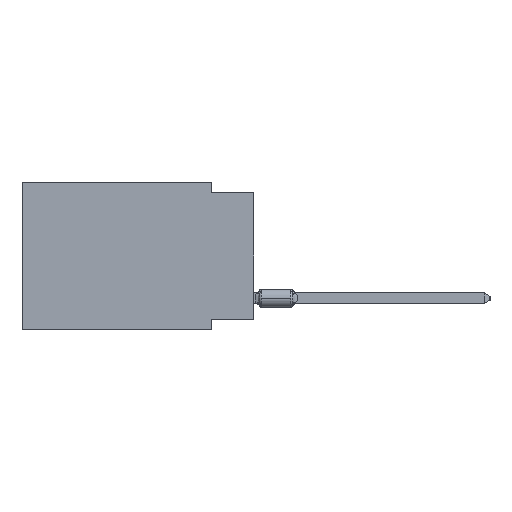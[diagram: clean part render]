
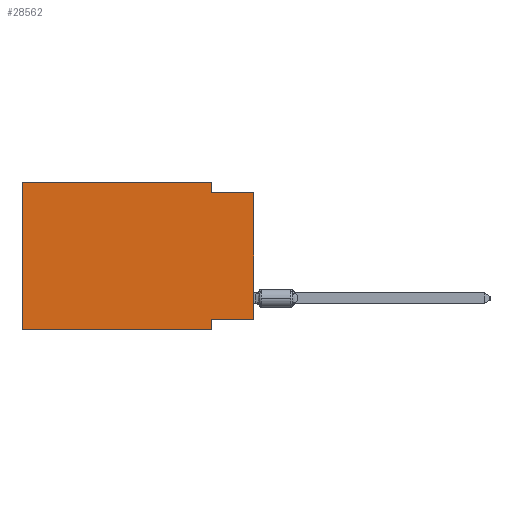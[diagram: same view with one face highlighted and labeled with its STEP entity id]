
A CAD part, left-side view. The second image highlights one B-rep face of the part: STEP entity #28562.
In plain terms, the highlighted planar face has unit normal (-1, 0, 0).
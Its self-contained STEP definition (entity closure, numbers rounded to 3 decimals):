
#42 = CARTESIAN_POINT ( 'NONE',  ( 0., 2.54, -8.89 ) ) ;
#937 = VECTOR ( 'NONE', #26357, 1000. ) ;
#982 = VECTOR ( 'NONE', #10857, 1000. ) ;
#1257 = EDGE_CURVE ( 'NONE', #8671, #54675, #59619, .T. ) ;
#1369 = LINE ( 'NONE', #26887, #47268 ) ;
#2557 = DIRECTION ( 'NONE',  ( 0., -1., 0. ) ) ;
#3318 = ORIENTED_EDGE ( 'NONE', *, *, #5943, .F. ) ;
#3636 = VERTEX_POINT ( 'NONE', #57415 ) ;
#4593 = CARTESIAN_POINT ( 'NONE',  ( 0., 2.54, 0. ) ) ;
#5943 = EDGE_CURVE ( 'NONE', #54675, #44059, #8694, .T. ) ;
#8671 = VERTEX_POINT ( 'NONE', #29459 ) ;
#8694 = LINE ( 'NONE', #29465, #54876 ) ;
#10195 = DIRECTION ( 'NONE',  ( 0., 1., 0. ) ) ;
#10857 = DIRECTION ( 'NONE',  ( 0., -1., 0. ) ) ;
#11293 = DIRECTION ( 'NONE',  ( 0., 0., 1. ) ) ;
#16132 = ORIENTED_EDGE ( 'NONE', *, *, #48546, .F. ) ;
#16175 = LINE ( 'NONE', #36650, #50894 ) ;
#16806 = DIRECTION ( 'NONE',  ( 0., 0., -1. ) ) ;
#19431 = VECTOR ( 'NONE', #11293, 1000. ) ;
#19963 = LINE ( 'NONE', #39179, #43681 ) ;
#20591 = CARTESIAN_POINT ( 'NONE',  ( 0., 2.54, -8.255 ) ) ;
#20739 = CARTESIAN_POINT ( 'NONE',  ( 0., 0., -8.255 ) ) ;
#21193 = AXIS2_PLACEMENT_3D ( 'NONE', #35976, #40442, #39469 ) ;
#21738 = CARTESIAN_POINT ( 'NONE',  ( 0., 13.97, -8.89 ) ) ;
#24330 = EDGE_LOOP ( 'NONE', ( #51633, #59758, #40295, #3318, #35253, #30114, #16132, #40734 ) ) ;
#25411 = PLANE ( 'NONE',  #21193 ) ;
#25545 = EDGE_CURVE ( 'NONE', #44059, #44435, #19963, .T. ) ;
#26357 = DIRECTION ( 'NONE',  ( 0., 0., 1. ) ) ;
#26548 = CARTESIAN_POINT ( 'NONE',  ( 0., 2.54, -0.635 ) ) ;
#26887 = CARTESIAN_POINT ( 'NONE',  ( 0., 0., -0.635 ) ) ;
#28562 = ADVANCED_FACE ( 'NONE', ( #44596 ), #25411, .F. ) ;
#29459 = CARTESIAN_POINT ( 'NONE',  ( 0., 13.97, -8.89 ) ) ;
#29465 = CARTESIAN_POINT ( 'NONE',  ( 0., 13.97, 0. ) ) ;
#29962 = VECTOR ( 'NONE', #10195, 1000. ) ;
#30114 = ORIENTED_EDGE ( 'NONE', *, *, #44304, .T. ) ;
#35253 = ORIENTED_EDGE ( 'NONE', *, *, #1257, .F. ) ;
#35976 = CARTESIAN_POINT ( 'NONE',  ( 0., 13.97, 0. ) ) ;
#36650 = CARTESIAN_POINT ( 'NONE',  ( 0., 2.54, -8.89 ) ) ;
#37870 = EDGE_CURVE ( 'NONE', #56214, #62409, #40573, .T. ) ;
#39179 = CARTESIAN_POINT ( 'NONE',  ( 0., 2.54, 0. ) ) ;
#39469 = DIRECTION ( 'NONE',  ( 0., 0., -1. ) ) ;
#40067 = CARTESIAN_POINT ( 'NONE',  ( 0., 0., -8.255 ) ) ;
#40295 = ORIENTED_EDGE ( 'NONE', *, *, #25545, .F. ) ;
#40442 = DIRECTION ( 'NONE',  ( 1., 0., 0. ) ) ;
#40573 = LINE ( 'NONE', #20739, #29962 ) ;
#40734 = ORIENTED_EDGE ( 'NONE', *, *, #37870, .F. ) ;
#42181 = CARTESIAN_POINT ( 'NONE',  ( 0., 13.97, 0. ) ) ;
#42943 = EDGE_CURVE ( 'NONE', #56214, #3636, #44541, .T. ) ;
#43681 = VECTOR ( 'NONE', #58987, 1000. ) ;
#44059 = VERTEX_POINT ( 'NONE', #4593 ) ;
#44304 = EDGE_CURVE ( 'NONE', #8671, #61014, #55639, .T. ) ;
#44435 = VERTEX_POINT ( 'NONE', #26548 ) ;
#44541 = LINE ( 'NONE', #44886, #19431 ) ;
#44596 = FACE_OUTER_BOUND ( 'NONE', #24330, .T. ) ;
#44886 = CARTESIAN_POINT ( 'NONE',  ( 0., 0., 0. ) ) ;
#47268 = VECTOR ( 'NONE', #2557, 1000. ) ;
#48546 = EDGE_CURVE ( 'NONE', #62409, #61014, #16175, .T. ) ;
#50894 = VECTOR ( 'NONE', #16806, 1000. ) ;
#51633 = ORIENTED_EDGE ( 'NONE', *, *, #42943, .T. ) ;
#54675 = VERTEX_POINT ( 'NONE', #42181 ) ;
#54876 = VECTOR ( 'NONE', #59522, 1000. ) ;
#55639 = LINE ( 'NONE', #21738, #982 ) ;
#56214 = VERTEX_POINT ( 'NONE', #40067 ) ;
#57415 = CARTESIAN_POINT ( 'NONE',  ( 0., 0., -0.635 ) ) ;
#58987 = DIRECTION ( 'NONE',  ( 0., 0., -1. ) ) ;
#59064 = EDGE_CURVE ( 'NONE', #44435, #3636, #1369, .T. ) ;
#59522 = DIRECTION ( 'NONE',  ( 0., -1., 0. ) ) ;
#59619 = LINE ( 'NONE', #60865, #937 ) ;
#59758 = ORIENTED_EDGE ( 'NONE', *, *, #59064, .F. ) ;
#60865 = CARTESIAN_POINT ( 'NONE',  ( 0., 13.97, 0. ) ) ;
#61014 = VERTEX_POINT ( 'NONE', #42 ) ;
#62409 = VERTEX_POINT ( 'NONE', #20591 ) ;
